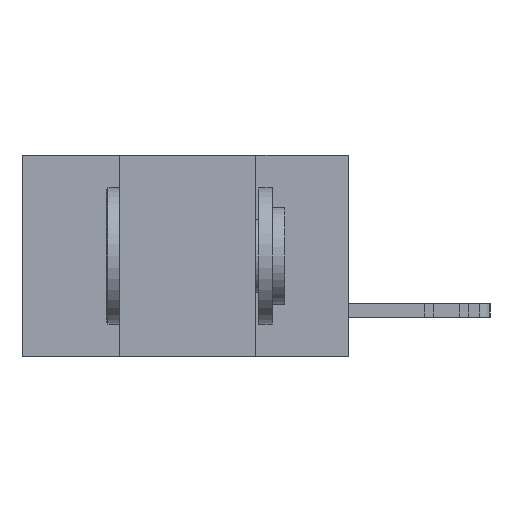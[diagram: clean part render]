
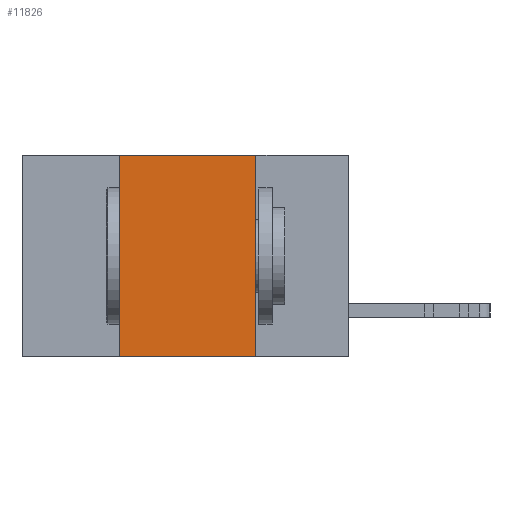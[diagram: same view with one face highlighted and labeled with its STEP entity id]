
A CAD part, left-side view. The second image highlights one B-rep face of the part: STEP entity #11826.
In plain terms, the highlighted planar face has unit normal (-1, 0, 0).
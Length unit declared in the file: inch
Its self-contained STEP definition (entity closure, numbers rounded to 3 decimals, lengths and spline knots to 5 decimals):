
#990 = ORIENTED_EDGE ( 'NONE', *, *, #2278, .F. ) ;
#1430 = ORIENTED_EDGE ( 'NONE', *, *, #19978, .T. ) ;
#1948 = EDGE_CURVE ( 'NONE', #8411, #12161, #22228, .T. ) ;
#2278 = EDGE_CURVE ( 'NONE', #3927, #8411, #23524, .T. ) ;
#3927 = VERTEX_POINT ( 'NONE', #6580 ) ;
#4001 = VECTOR ( 'NONE', #9381, 39.37008 ) ;
#5059 = CARTESIAN_POINT ( 'NONE',  ( 0., 0.17, 0. ) ) ;
#6030 = VECTOR ( 'NONE', #25462, 39.37008 ) ;
#6102 = DIRECTION ( 'NONE',  ( 0., 0., -1. ) ) ;
#6580 = CARTESIAN_POINT ( 'NONE',  ( 0., 0.42, -0.37 ) ) ;
#6768 = FACE_OUTER_BOUND ( 'NONE', #8076, .T. ) ;
#8076 = EDGE_LOOP ( 'NONE', ( #20485, #23340, #990, #1430 ) ) ;
#8083 = DIRECTION ( 'NONE',  ( 0., 0., -1. ) ) ;
#8411 = VERTEX_POINT ( 'NONE', #22585 ) ;
#8697 = EDGE_CURVE ( 'NONE', #12161, #24078, #21110, .T. ) ;
#9289 = CARTESIAN_POINT ( 'NONE',  ( 0., 0.6, 0. ) ) ;
#9381 = DIRECTION ( 'NONE',  ( 0., -1., 0. ) ) ;
#9582 = CARTESIAN_POINT ( 'NONE',  ( 0., 0.6, -0.37 ) ) ;
#10284 = CARTESIAN_POINT ( 'NONE',  ( 0., 0.17, 0. ) ) ;
#11826 = ADVANCED_FACE ( 'NONE', ( #6768 ), #21398, .F. ) ;
#12161 = VERTEX_POINT ( 'NONE', #5059 ) ;
#14559 = VECTOR ( 'NONE', #8083, 39.37008 ) ;
#16208 = VECTOR ( 'NONE', #22750, 39.37008 ) ;
#17109 = CARTESIAN_POINT ( 'NONE',  ( 0., 0.6, 0. ) ) ;
#17807 = AXIS2_PLACEMENT_3D ( 'NONE', #17109, #19323, #6102 ) ;
#19323 = DIRECTION ( 'NONE',  ( 1., 0., 0. ) ) ;
#19978 = EDGE_CURVE ( 'NONE', #3927, #24078, #22036, .T. ) ;
#20485 = ORIENTED_EDGE ( 'NONE', *, *, #8697, .F. ) ;
#21110 = LINE ( 'NONE', #10284, #14559 ) ;
#21398 = PLANE ( 'NONE',  #17807 ) ;
#22036 = LINE ( 'NONE', #9582, #16208 ) ;
#22087 = CARTESIAN_POINT ( 'NONE',  ( 0., 0.42, 0. ) ) ;
#22228 = LINE ( 'NONE', #9289, #4001 ) ;
#22585 = CARTESIAN_POINT ( 'NONE',  ( 0., 0.42, 0. ) ) ;
#22750 = DIRECTION ( 'NONE',  ( 0., -1., 0. ) ) ;
#23340 = ORIENTED_EDGE ( 'NONE', *, *, #1948, .F. ) ;
#23524 = LINE ( 'NONE', #22087, #6030 ) ;
#24078 = VERTEX_POINT ( 'NONE', #26143 ) ;
#25462 = DIRECTION ( 'NONE',  ( 0., 0., 1. ) ) ;
#26143 = CARTESIAN_POINT ( 'NONE',  ( 0., 0.17, -0.37 ) ) ;
